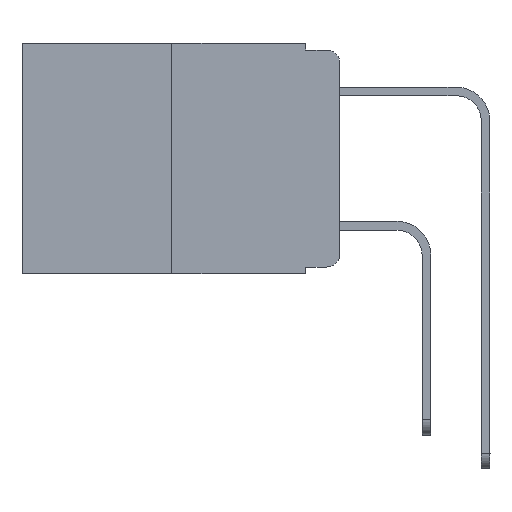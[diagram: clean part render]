
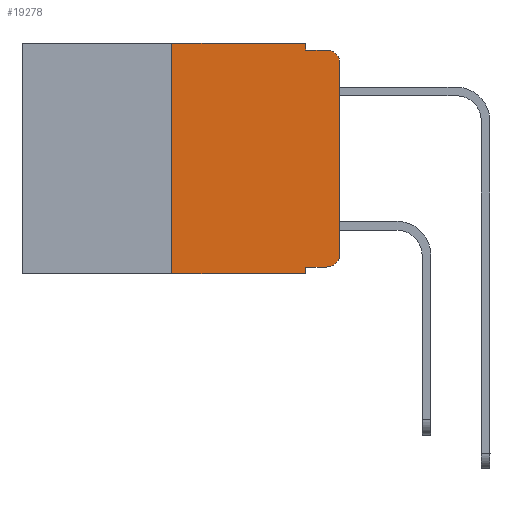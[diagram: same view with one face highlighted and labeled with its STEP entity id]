
A CAD part, left-side view. The second image highlights one B-rep face of the part: STEP entity #19278.
In plain terms, the highlighted planar face has unit normal (-1, 0, 0).
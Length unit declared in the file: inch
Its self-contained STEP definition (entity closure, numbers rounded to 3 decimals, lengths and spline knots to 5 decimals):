
#182 = CARTESIAN_POINT ( 'NONE',  ( 0., 0.25, -0.343 ) ) ;
#226 = VECTOR ( 'NONE', #24590, 39.37008 ) ;
#861 = CARTESIAN_POINT ( 'NONE',  ( 0., 0.051, -0.333 ) ) ;
#1649 = CARTESIAN_POINT ( 'NONE',  ( 0., 0.25, 0. ) ) ;
#1864 = VERTEX_POINT ( 'NONE', #26178 ) ;
#2232 = EDGE_CURVE ( 'NONE', #13819, #14727, #15342, .T. ) ;
#2343 = EDGE_CURVE ( 'NONE', #9212, #11758, #20532, .T. ) ;
#2427 = DIRECTION ( 'NONE',  ( 0., 0., -1. ) ) ;
#2444 = VERTEX_POINT ( 'NONE', #11538 ) ;
#3670 = DIRECTION ( 'NONE',  ( 1., 0., 0. ) ) ;
#3852 = CIRCLE ( 'NONE', #10119, 0.02 ) ;
#4151 = EDGE_CURVE ( 'NONE', #7655, #9212, #5759, .T. ) ;
#4496 = EDGE_CURVE ( 'NONE', #15105, #1864, #22033, .T. ) ;
#4632 = CARTESIAN_POINT ( 'NONE',  ( 0., 0.051, -0.333 ) ) ;
#5112 = EDGE_CURVE ( 'NONE', #12236, #7655, #17072, .T. ) ;
#5144 = ORIENTED_EDGE ( 'NONE', *, *, #2343, .F. ) ;
#5360 = DIRECTION ( 'NONE',  ( 0., 0., -1. ) ) ;
#5367 = DIRECTION ( 'NONE',  ( 0., 0., -1. ) ) ;
#5505 = CARTESIAN_POINT ( 'NONE',  ( 0., 0.051, 0. ) ) ;
#5550 = ORIENTED_EDGE ( 'NONE', *, *, #8244, .F. ) ;
#5659 = VECTOR ( 'NONE', #10972, 39.37008 ) ;
#5710 = DIRECTION ( 'NONE',  ( 0., 0., -1. ) ) ;
#5759 = LINE ( 'NONE', #18818, #11887 ) ;
#5915 = ORIENTED_EDGE ( 'NONE', *, *, #17806, .T. ) ;
#6034 = DIRECTION ( 'NONE',  ( 0., -1., 0. ) ) ;
#6165 = CARTESIAN_POINT ( 'NONE',  ( 0., 0., 0. ) ) ;
#6374 = DIRECTION ( 'NONE',  ( 0., -1., 0. ) ) ;
#7062 = VECTOR ( 'NONE', #9842, 39.37008 ) ;
#7261 = CARTESIAN_POINT ( 'NONE',  ( 0., 0.02, -0.03 ) ) ;
#7319 = CARTESIAN_POINT ( 'NONE',  ( 0., 0.051, 0. ) ) ;
#7386 = CARTESIAN_POINT ( 'NONE',  ( 0., 0., -0.313 ) ) ;
#7655 = VERTEX_POINT ( 'NONE', #20366 ) ;
#8244 = EDGE_CURVE ( 'NONE', #11758, #1864, #23657, .T. ) ;
#8365 = DIRECTION ( 'NONE',  ( -1., 0., 0. ) ) ;
#8418 = ORIENTED_EDGE ( 'NONE', *, *, #4496, .T. ) ;
#9052 = EDGE_CURVE ( 'NONE', #13819, #2444, #18415, .T. ) ;
#9212 = VERTEX_POINT ( 'NONE', #5505 ) ;
#9842 = DIRECTION ( 'NONE',  ( 0., 0., 1. ) ) ;
#10119 = AXIS2_PLACEMENT_3D ( 'NONE', #10465, #8365, #5710 ) ;
#10457 = CARTESIAN_POINT ( 'NONE',  ( 0., 0.051, -0.01 ) ) ;
#10465 = CARTESIAN_POINT ( 'NONE',  ( 0., 0.02, -0.313 ) ) ;
#10972 = DIRECTION ( 'NONE',  ( 0., -1., 0. ) ) ;
#11538 = CARTESIAN_POINT ( 'NONE',  ( 0., 0.02, -0.333 ) ) ;
#11758 = VERTEX_POINT ( 'NONE', #21838 ) ;
#11887 = VECTOR ( 'NONE', #6034, 39.37008 ) ;
#12118 = VECTOR ( 'NONE', #2427, 39.37008 ) ;
#12157 = AXIS2_PLACEMENT_3D ( 'NONE', #7261, #15835, #22431 ) ;
#12236 = VERTEX_POINT ( 'NONE', #182 ) ;
#13819 = VERTEX_POINT ( 'NONE', #4632 ) ;
#14158 = ORIENTED_EDGE ( 'NONE', *, *, #2232, .F. ) ;
#14727 = VERTEX_POINT ( 'NONE', #19591 ) ;
#15105 = VERTEX_POINT ( 'NONE', #21372 ) ;
#15342 = LINE ( 'NONE', #21655, #12118 ) ;
#15835 = DIRECTION ( 'NONE',  ( -1., 0., 0. ) ) ;
#17072 = LINE ( 'NONE', #1649, #19857 ) ;
#17806 = EDGE_CURVE ( 'NONE', #12236, #14727, #20101, .T. ) ;
#17851 = ORIENTED_EDGE ( 'NONE', *, *, #5112, .F. ) ;
#18415 = LINE ( 'NONE', #861, #226 ) ;
#18425 = VECTOR ( 'NONE', #5367, 39.37008 ) ;
#18703 = FACE_OUTER_BOUND ( 'NONE', #22435, .T. ) ;
#18818 = CARTESIAN_POINT ( 'NONE',  ( 0., 0.473, 0. ) ) ;
#18985 = EDGE_CURVE ( 'NONE', #2444, #21739, #3852, .T. ) ;
#19032 = ORIENTED_EDGE ( 'NONE', *, *, #4151, .F. ) ;
#19135 = ORIENTED_EDGE ( 'NONE', *, *, #18985, .T. ) ;
#19278 = ADVANCED_FACE ( 'NONE', ( #18703 ), #20383, .F. ) ;
#19315 = VECTOR ( 'NONE', #6374, 39.37008 ) ;
#19591 = CARTESIAN_POINT ( 'NONE',  ( 0., 0.051, -0.343 ) ) ;
#19857 = VECTOR ( 'NONE', #20887, 39.37008 ) ;
#20101 = LINE ( 'NONE', #23912, #5659 ) ;
#20366 = CARTESIAN_POINT ( 'NONE',  ( 0., 0.25, 0. ) ) ;
#20383 = PLANE ( 'NONE',  #27623 ) ;
#20532 = LINE ( 'NONE', #7319, #18425 ) ;
#20887 = DIRECTION ( 'NONE',  ( 0., 0., 1. ) ) ;
#21075 = EDGE_CURVE ( 'NONE', #21739, #15105, #21313, .T. ) ;
#21313 = LINE ( 'NONE', #6165, #7062 ) ;
#21372 = CARTESIAN_POINT ( 'NONE',  ( 0., 0., -0.03 ) ) ;
#21655 = CARTESIAN_POINT ( 'NONE',  ( 0., 0.051, 0. ) ) ;
#21739 = VERTEX_POINT ( 'NONE', #7386 ) ;
#21838 = CARTESIAN_POINT ( 'NONE',  ( 0., 0.051, -0.01 ) ) ;
#22033 = CIRCLE ( 'NONE', #12157, 0.02 ) ;
#22431 = DIRECTION ( 'NONE',  ( 0., 0., -1. ) ) ;
#22435 = EDGE_LOOP ( 'NONE', ( #24907, #8418, #5550, #5144, #19032, #17851, #5915, #14158, #22805, #19135 ) ) ;
#22805 = ORIENTED_EDGE ( 'NONE', *, *, #9052, .T. ) ;
#23657 = LINE ( 'NONE', #10457, #19315 ) ;
#23912 = CARTESIAN_POINT ( 'NONE',  ( 0., 0.473, -0.343 ) ) ;
#24590 = DIRECTION ( 'NONE',  ( 0., -1., 0. ) ) ;
#24907 = ORIENTED_EDGE ( 'NONE', *, *, #21075, .T. ) ;
#26178 = CARTESIAN_POINT ( 'NONE',  ( 0., 0.02, -0.01 ) ) ;
#27263 = CARTESIAN_POINT ( 'NONE',  ( 0., 0.473, 0. ) ) ;
#27623 = AXIS2_PLACEMENT_3D ( 'NONE', #27263, #3670, #5360 ) ;
